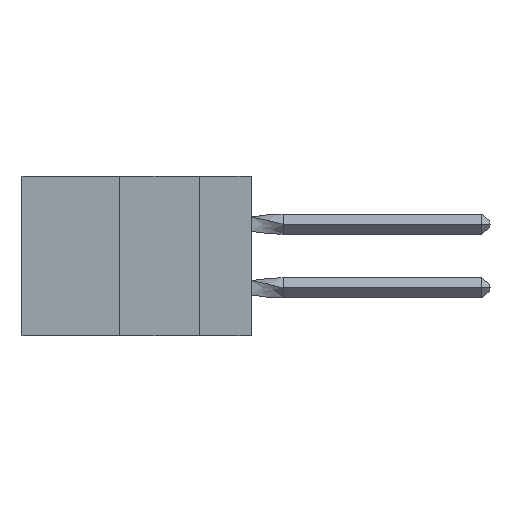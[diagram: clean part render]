
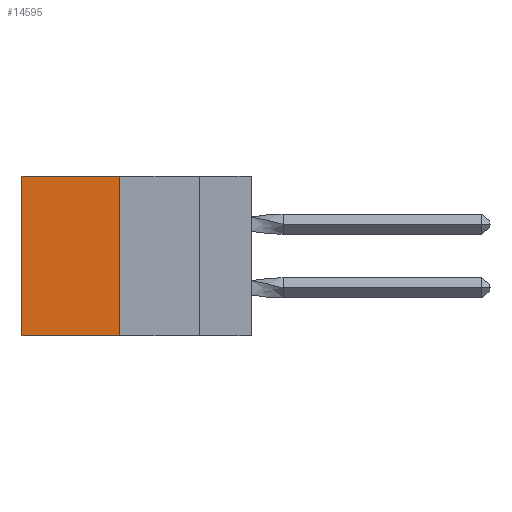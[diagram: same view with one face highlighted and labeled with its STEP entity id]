
A CAD part, left-side view. The second image highlights one B-rep face of the part: STEP entity #14595.
In plain terms, the highlighted planar face has unit normal (-1, 0, 0).
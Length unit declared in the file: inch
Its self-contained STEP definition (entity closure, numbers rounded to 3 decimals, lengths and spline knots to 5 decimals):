
#470 = EDGE_CURVE ( 'NONE', #11717, #9531, #11245, .T. ) ;
#685 = LINE ( 'NONE', #3498, #8580 ) ;
#751 = LINE ( 'NONE', #13877, #12612 ) ;
#805 = DIRECTION ( 'NONE',  ( 0., 1., 0. ) ) ;
#870 = VERTEX_POINT ( 'NONE', #12814 ) ;
#967 = PLANE ( 'NONE',  #10082 ) ;
#2116 = VECTOR ( 'NONE', #2885, 39.37008 ) ;
#2561 = ORIENTED_EDGE ( 'NONE', *, *, #7262, .T. ) ;
#2885 = DIRECTION ( 'NONE',  ( 0., 1., 0. ) ) ;
#3498 = CARTESIAN_POINT ( 'NONE',  ( 0.305, 0.413, -0.5 ) ) ;
#3521 = VECTOR ( 'NONE', #15337, 39.37008 ) ;
#4475 = CARTESIAN_POINT ( 'NONE',  ( 0.305, 0.72, 0. ) ) ;
#4779 = DIRECTION ( 'NONE',  ( 1., 0., 0. ) ) ;
#5427 = CARTESIAN_POINT ( 'NONE',  ( 0.305, 0.413, -0.5 ) ) ;
#5493 = LINE ( 'NONE', #15357, #2116 ) ;
#5777 = ORIENTED_EDGE ( 'NONE', *, *, #7137, .T. ) ;
#7137 = EDGE_CURVE ( 'NONE', #13830, #870, #751, .T. ) ;
#7262 = EDGE_CURVE ( 'NONE', #11717, #13830, #5493, .T. ) ;
#8580 = VECTOR ( 'NONE', #805, 39.37008 ) ;
#9017 = CARTESIAN_POINT ( 'NONE',  ( 0.305, 0.413, -0.5 ) ) ;
#9084 = EDGE_CURVE ( 'NONE', #9531, #870, #685, .T. ) ;
#9531 = VERTEX_POINT ( 'NONE', #5427 ) ;
#10082 = AXIS2_PLACEMENT_3D ( 'NONE', #12509, #4779, #12451 ) ;
#10279 = DIRECTION ( 'NONE',  ( 0., 0., -1. ) ) ;
#10541 = ORIENTED_EDGE ( 'NONE', *, *, #9084, .F. ) ;
#11245 = LINE ( 'NONE', #9017, #3521 ) ;
#11717 = VERTEX_POINT ( 'NONE', #14657 ) ;
#12451 = DIRECTION ( 'NONE',  ( 0., 0., -1. ) ) ;
#12509 = CARTESIAN_POINT ( 'NONE',  ( 0.305, 0.413, -0.5 ) ) ;
#12612 = VECTOR ( 'NONE', #10279, 39.37008 ) ;
#12814 = CARTESIAN_POINT ( 'NONE',  ( 0.305, 0.72, -0.5 ) ) ;
#13830 = VERTEX_POINT ( 'NONE', #4475 ) ;
#13877 = CARTESIAN_POINT ( 'NONE',  ( 0.305, 0.72, -0.5 ) ) ;
#14358 = EDGE_LOOP ( 'NONE', ( #5777, #10541, #14988, #2561 ) ) ;
#14595 = ADVANCED_FACE ( 'NONE', ( #16120 ), #967, .F. ) ;
#14657 = CARTESIAN_POINT ( 'NONE',  ( 0.305, 0.413, 0. ) ) ;
#14988 = ORIENTED_EDGE ( 'NONE', *, *, #470, .F. ) ;
#15337 = DIRECTION ( 'NONE',  ( 0., 0., -1. ) ) ;
#15357 = CARTESIAN_POINT ( 'NONE',  ( 0.305, 0.413, 0. ) ) ;
#16120 = FACE_OUTER_BOUND ( 'NONE', #14358, .T. ) ;
